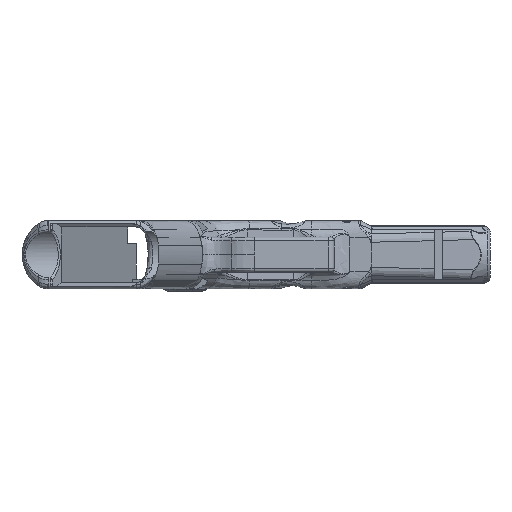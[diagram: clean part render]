
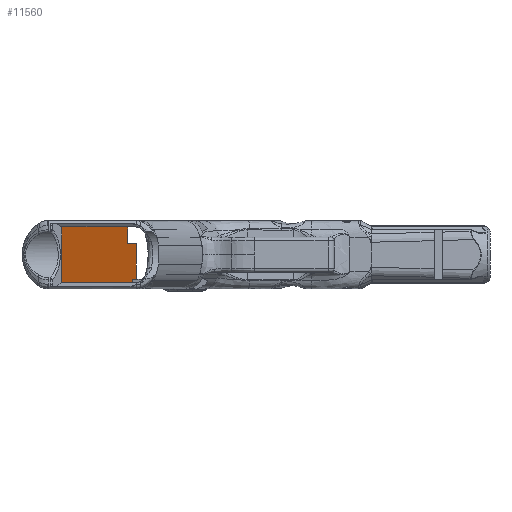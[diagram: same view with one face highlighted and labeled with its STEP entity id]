
A CAD part, front view. The second image highlights one B-rep face of the part: STEP entity #11560.
In plain terms, the highlighted planar face has unit normal (0.951, -0.309, 0).
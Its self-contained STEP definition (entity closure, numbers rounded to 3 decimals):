
#1050=ELLIPSE('',#12144,1.051,1.);
#1060=ELLIPSE('',#12171,1.051,1.);
#1775=FACE_OUTER_BOUND('',#2417,.T.);
#2417=EDGE_LOOP('',(#10256,#10257,#10258,#10259,#10260,#10261,#10262,#10263,
#10264,#10265));
#3259=LINE('',#27382,#3909);
#3363=LINE('',#30789,#4013);
#3376=LINE('',#31247,#4026);
#3497=LINE('',#42662,#4147);
#3520=LINE('',#44008,#4170);
#3523=LINE('',#44316,#4173);
#3529=LINE('',#44928,#4179);
#3530=LINE('',#44929,#4180);
#3909=VECTOR('',#13529,10.);
#4013=VECTOR('',#13965,10.);
#4026=VECTOR('',#14006,10.);
#4147=VECTOR('',#14565,10.);
#4170=VECTOR('',#14684,10.);
#4173=VECTOR('',#14693,10.);
#4179=VECTOR('',#14729,10.);
#4180=VECTOR('',#14730,10.);
#4822=VERTEX_POINT('',#27379);
#4823=VERTEX_POINT('',#27381);
#4951=VERTEX_POINT('',#29740);
#4992=VERTEX_POINT('',#30769);
#4994=VERTEX_POINT('',#30773);
#5000=VERTEX_POINT('',#30787);
#5308=VERTEX_POINT('',#42660);
#5337=VERTEX_POINT('',#44006);
#5344=VERTEX_POINT('',#44313);
#5345=VERTEX_POINT('',#44315);
#6198=EDGE_CURVE('',#4823,#4822,#3259,.T.);
#6402=EDGE_CURVE('',#4951,#4822,#1050,.F.);
#6461=EDGE_CURVE('',#4994,#4992,#1060,.F.);
#6468=EDGE_CURVE('',#4994,#5000,#3363,.T.);
#6500=EDGE_CURVE('',#4992,#4951,#3376,.F.);
#6984=EDGE_CURVE('',#5308,#5000,#3497,.T.);
#7048=EDGE_CURVE('',#5337,#5308,#3520,.T.);
#7057=EDGE_CURVE('',#5344,#5345,#3523,.T.);
#7074=EDGE_CURVE('',#5345,#5337,#3529,.T.);
#7075=EDGE_CURVE('',#4823,#5344,#3530,.T.);
#10256=ORIENTED_EDGE('',*,*,#6198,.T.);
#10257=ORIENTED_EDGE('',*,*,#6402,.F.);
#10258=ORIENTED_EDGE('',*,*,#6500,.F.);
#10259=ORIENTED_EDGE('',*,*,#6461,.F.);
#10260=ORIENTED_EDGE('',*,*,#6468,.T.);
#10261=ORIENTED_EDGE('',*,*,#6984,.F.);
#10262=ORIENTED_EDGE('',*,*,#7048,.F.);
#10263=ORIENTED_EDGE('',*,*,#7074,.F.);
#10264=ORIENTED_EDGE('',*,*,#7057,.F.);
#10265=ORIENTED_EDGE('',*,*,#7075,.F.);
#11019=PLANE('',#12471);
#11560=ADVANCED_FACE('',(#1775),#11019,.F.);
#12144=AXIS2_PLACEMENT_3D('',#29741,#13894,#13895);
#12171=AXIS2_PLACEMENT_3D('',#30775,#13955,#13956);
#12471=AXIS2_PLACEMENT_3D('',#44927,#14727,#14728);
#13529=DIRECTION('',(-0.309,-0.951,0.));
#13894=DIRECTION('center_axis',(-0.951,0.309,0.));
#13895=DIRECTION('ref_axis',(-0.309,-0.951,0.));
#13955=DIRECTION('center_axis',(-0.951,0.309,0.));
#13956=DIRECTION('ref_axis',(-0.309,-0.951,0.));
#13965=DIRECTION('',(0.309,0.951,0.));
#14006=DIRECTION('',(0.,0.,-1.));
#14565=DIRECTION('',(0.,0.,-1.));
#14684=DIRECTION('',(-0.309,-0.951,0.));
#14693=DIRECTION('',(0.309,0.951,0.));
#14727=DIRECTION('center_axis',(-0.951,0.309,0.));
#14728=DIRECTION('ref_axis',(0.,0.,
1.));
#14729=DIRECTION('',(0.,0.,-1.));
#14730=DIRECTION('',(0.,0.,-1.));
#27379=CARTESIAN_POINT('',(2.294,-97.822,11.75));
#27381=CARTESIAN_POINT('',(30.049,-12.4,11.75));
#27382=CARTESIAN_POINT('',(2.312,-97.765,11.75));
#29740=CARTESIAN_POINT('',(2.236,-98.,11.766));
#29741=CARTESIAN_POINT('Origin',(2.294,-97.822,12.75));
#30769=CARTESIAN_POINT('',(2.236,-98.,-11.766));
#30773=CARTESIAN_POINT('',(2.294,-97.822,-11.75));
#30775=CARTESIAN_POINT('Origin',(2.294,-97.822,-12.75));
#30787=CARTESIAN_POINT('',(32.169,-5.875,-11.75));
#30789=CARTESIAN_POINT('',(2.312,-97.765,-11.75));
#31247=CARTESIAN_POINT('',(2.236,-98.,-18.375));
#42660=CARTESIAN_POINT('',(32.169,-5.875,-10.375));
#42662=CARTESIAN_POINT('',(32.169,-5.875,-5.875));
#44006=CARTESIAN_POINT('',(33.591,-1.5,-10.375));
#44008=CARTESIAN_POINT('',(17.241,-51.82,-10.375));
#44313=CARTESIAN_POINT('',(30.049,-12.4,4.75));
#44315=CARTESIAN_POINT('',(33.591,-1.5,4.75));
#44316=CARTESIAN_POINT('',(18.86,-46.836,4.75));
#44927=CARTESIAN_POINT('Origin',(2.312,-97.765,-11.75));
#44928=CARTESIAN_POINT('',(33.591,-1.5,-5.875));
#44929=CARTESIAN_POINT('',(30.049,-12.4,2.982));
